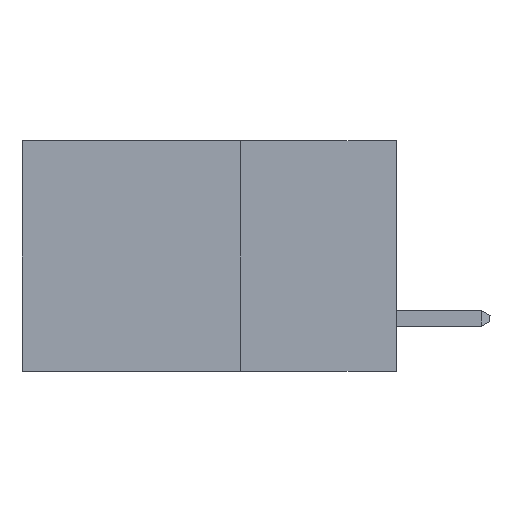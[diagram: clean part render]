
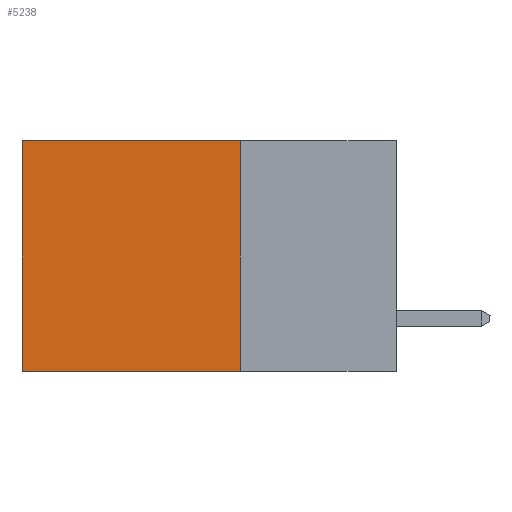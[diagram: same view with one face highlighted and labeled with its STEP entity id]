
A CAD part, left-side view. The second image highlights one B-rep face of the part: STEP entity #5238.
In plain terms, the highlighted planar face has unit normal (-1, 0, 0).
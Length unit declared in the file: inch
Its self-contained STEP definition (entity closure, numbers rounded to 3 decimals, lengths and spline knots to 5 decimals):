
#612 = ORIENTED_EDGE ( 'NONE', *, *, #1337, .T. ) ;
#1074 = LINE ( 'NONE', #18672, #11050 ) ;
#1337 = EDGE_CURVE ( 'NONE', #22558, #18002, #20401, .T. ) ;
#1361 = CARTESIAN_POINT ( 'NONE',  ( 0.2615, 0.6, -0.37 ) ) ;
#1375 = EDGE_LOOP ( 'NONE', ( #612, #5643, #2958, #4838 ) ) ;
#2827 = VECTOR ( 'NONE', #24611, 39.37008 ) ;
#2886 = DIRECTION ( 'NONE',  ( 0., 0., -1. ) ) ;
#2958 = ORIENTED_EDGE ( 'NONE', *, *, #11730, .F. ) ;
#4808 = PLANE ( 'NONE',  #18554 ) ;
#4838 = ORIENTED_EDGE ( 'NONE', *, *, #8000, .T. ) ;
#5238 = ADVANCED_FACE ( 'NONE', ( #12937 ), #4808, .F. ) ;
#5327 = LINE ( 'NONE', #25473, #11265 ) ;
#5643 = ORIENTED_EDGE ( 'NONE', *, *, #19839, .F. ) ;
#7596 = CARTESIAN_POINT ( 'NONE',  ( 0.2615, 0.25, -0.37 ) ) ;
#8000 = EDGE_CURVE ( 'NONE', #9109, #22558, #18733, .T. ) ;
#9109 = VERTEX_POINT ( 'NONE', #22417 ) ;
#10781 = CARTESIAN_POINT ( 'NONE',  ( 0.2615, 0.25, 0. ) ) ;
#11050 = VECTOR ( 'NONE', #20626, 39.37008 ) ;
#11265 = VECTOR ( 'NONE', #11644, 39.37008 ) ;
#11644 = DIRECTION ( 'NONE',  ( 0., 1., 0. ) ) ;
#11730 = EDGE_CURVE ( 'NONE', #9109, #20839, #1074, .T. ) ;
#12937 = FACE_OUTER_BOUND ( 'NONE', #1375, .T. ) ;
#14819 = DIRECTION ( 'NONE',  ( 1., 0., 0. ) ) ;
#17807 = CARTESIAN_POINT ( 'NONE',  ( 0.2615, 0.6, 0. ) ) ;
#18002 = VERTEX_POINT ( 'NONE', #23554 ) ;
#18554 = AXIS2_PLACEMENT_3D ( 'NONE', #24656, #14819, #2886 ) ;
#18672 = CARTESIAN_POINT ( 'NONE',  ( 0.2615, 0.25, -0.37 ) ) ;
#18733 = LINE ( 'NONE', #10781, #2827 ) ;
#19839 = EDGE_CURVE ( 'NONE', #20839, #18002, #5327, .T. ) ;
#20401 = LINE ( 'NONE', #1361, #24401 ) ;
#20626 = DIRECTION ( 'NONE',  ( 0., 0., -1. ) ) ;
#20839 = VERTEX_POINT ( 'NONE', #7596 ) ;
#22004 = DIRECTION ( 'NONE',  ( 0., 0., -1. ) ) ;
#22417 = CARTESIAN_POINT ( 'NONE',  ( 0.2615, 0.25, 0. ) ) ;
#22558 = VERTEX_POINT ( 'NONE', #17807 ) ;
#23554 = CARTESIAN_POINT ( 'NONE',  ( 0.2615, 0.6, -0.37 ) ) ;
#24401 = VECTOR ( 'NONE', #22004, 39.37008 ) ;
#24611 = DIRECTION ( 'NONE',  ( 0., 1., 0. ) ) ;
#24656 = CARTESIAN_POINT ( 'NONE',  ( 0.2615, 0.25, -0.37 ) ) ;
#25473 = CARTESIAN_POINT ( 'NONE',  ( 0.2615, 0.25, -0.37 ) ) ;
